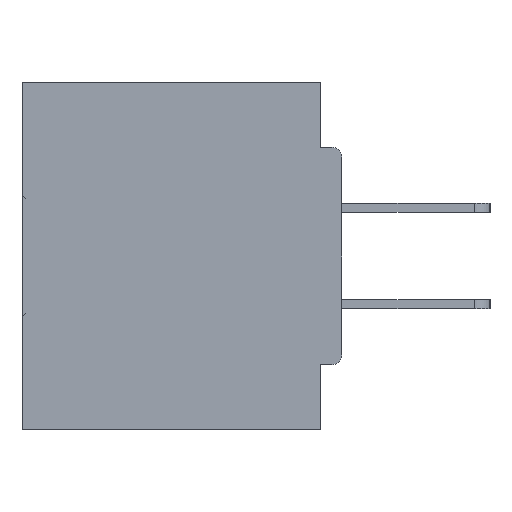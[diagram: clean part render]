
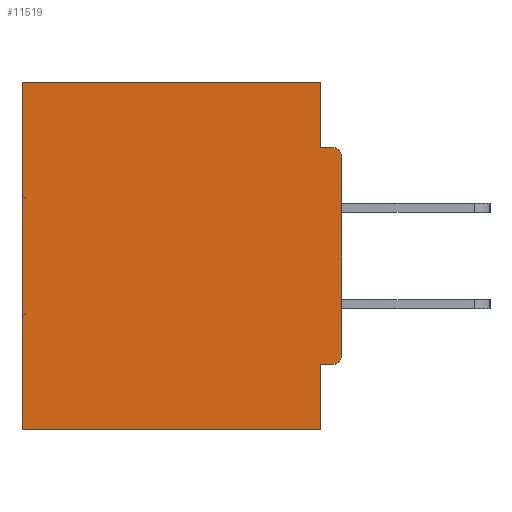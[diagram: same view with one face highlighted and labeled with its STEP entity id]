
A CAD part, left-side view. The second image highlights one B-rep face of the part: STEP entity #11519.
In plain terms, the highlighted planar face has unit normal (-1, 0, 0).
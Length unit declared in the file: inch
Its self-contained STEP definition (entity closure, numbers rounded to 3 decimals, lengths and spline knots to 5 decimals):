
#650 = DIRECTION ( 'NONE',  ( 0., 0., -1. ) ) ;
#1674 = CARTESIAN_POINT ( 'NONE',  ( 0.298, 0.031, -0.5 ) ) ;
#2309 = DIRECTION ( 'NONE',  ( 0., 0., -1. ) ) ;
#2411 = CARTESIAN_POINT ( 'NONE',  ( 0.298, 0.031, -0.5 ) ) ;
#2700 = VECTOR ( 'NONE', #34223, 39.37008 ) ;
#2734 = EDGE_CURVE ( 'NONE', #3310, #17542, #43901, .T. ) ;
#2821 = VECTOR ( 'NONE', #18981, 39.37008 ) ;
#2881 = ORIENTED_EDGE ( 'NONE', *, *, #22470, .F. ) ;
#3310 = VERTEX_POINT ( 'NONE', #43236 ) ;
#4273 = VERTEX_POINT ( 'NONE', #42371 ) ;
#4668 = ORIENTED_EDGE ( 'NONE', *, *, #32894, .F. ) ;
#4738 = VECTOR ( 'NONE', #2309, 39.37008 ) ;
#4815 = CARTESIAN_POINT ( 'NONE',  ( 0.298, 0., 0. ) ) ;
#5867 = CIRCLE ( 'NONE', #31879, 0.015 ) ;
#6453 = ORIENTED_EDGE ( 'NONE', *, *, #44425, .F. ) ;
#6900 = LINE ( 'NONE', #30315, #4738 ) ;
#7032 = DIRECTION ( 'NONE',  ( 0., 0., -1. ) ) ;
#7067 = CARTESIAN_POINT ( 'NONE',  ( 0.298, 0., -0.0935 ) ) ;
#7147 = VERTEX_POINT ( 'NONE', #1674 ) ;
#8447 = DIRECTION ( 'NONE',  ( 0., 0., -1. ) ) ;
#9360 = EDGE_CURVE ( 'NONE', #7147, #17542, #41419, .T. ) ;
#10008 = CARTESIAN_POINT ( 'NONE',  ( 0.298, 0., -0.3915 ) ) ;
#10308 = CARTESIAN_POINT ( 'NONE',  ( 0.298, 0.46, -0.5 ) ) ;
#10329 = CARTESIAN_POINT ( 'NONE',  ( 0.298, 0.015, -0.4065 ) ) ;
#10981 = VERTEX_POINT ( 'NONE', #10329 ) ;
#11519 = ADVANCED_FACE ( 'NONE', ( #39251 ), #18842, .F. ) ;
#11791 = CARTESIAN_POINT ( 'NONE',  ( 0.298, 0.015, -0.1085 ) ) ;
#11940 = EDGE_CURVE ( 'NONE', #10981, #24321, #34385, .T. ) ;
#13365 = DIRECTION ( 'NONE',  ( 0., 1., 0. ) ) ;
#14458 = ORIENTED_EDGE ( 'NONE', *, *, #2734, .T. ) ;
#15393 = ORIENTED_EDGE ( 'NONE', *, *, #26734, .F. ) ;
#15981 = ORIENTED_EDGE ( 'NONE', *, *, #9360, .F. ) ;
#16118 = AXIS2_PLACEMENT_3D ( 'NONE', #21905, #42683, #29031 ) ;
#16485 = CARTESIAN_POINT ( 'NONE',  ( 0.298, 0.031, -0.0935 ) ) ;
#17542 = VERTEX_POINT ( 'NONE', #10308 ) ;
#18842 = PLANE ( 'NONE',  #16118 ) ;
#18981 = DIRECTION ( 'NONE',  ( 0., 1., 0. ) ) ;
#21098 = DIRECTION ( 'NONE',  ( 0., -1., 0. ) ) ;
#21227 = LINE ( 'NONE', #2411, #2700 ) ;
#21905 = CARTESIAN_POINT ( 'NONE',  ( 0.298, 0., 0. ) ) ;
#22470 = EDGE_CURVE ( 'NONE', #24321, #7147, #21227, .T. ) ;
#22751 = DIRECTION ( 'NONE',  ( 0., 1., 0. ) ) ;
#22793 = VECTOR ( 'NONE', #21098, 39.37008 ) ;
#23067 = CARTESIAN_POINT ( 'NONE',  ( 0.298, 0., -0.5 ) ) ;
#23144 = EDGE_CURVE ( 'NONE', #32583, #4273, #37032, .T. ) ;
#24321 = VERTEX_POINT ( 'NONE', #33724 ) ;
#24850 = CARTESIAN_POINT ( 'NONE',  ( 0.298, 0.46, 0. ) ) ;
#25081 = VECTOR ( 'NONE', #13365, 39.37008 ) ;
#25689 = VECTOR ( 'NONE', #22751, 39.37008 ) ;
#26417 = DIRECTION ( 'NONE',  ( -1., 0., 0. ) ) ;
#26734 = EDGE_CURVE ( 'NONE', #43732, #31339, #6900, .T. ) ;
#27006 = VECTOR ( 'NONE', #650, 39.37008 ) ;
#27881 = ORIENTED_EDGE ( 'NONE', *, *, #41100, .T. ) ;
#29031 = DIRECTION ( 'NONE',  ( 0., 0., -1. ) ) ;
#30315 = CARTESIAN_POINT ( 'NONE',  ( 0.298, 0.031, -0.5 ) ) ;
#31339 = VERTEX_POINT ( 'NONE', #16485 ) ;
#31353 = AXIS2_PLACEMENT_3D ( 'NONE', #11791, #36349, #36644 ) ;
#31879 = AXIS2_PLACEMENT_3D ( 'NONE', #36483, #26417, #8447 ) ;
#32151 = CARTESIAN_POINT ( 'NONE',  ( 0.298, 0., -0.1085 ) ) ;
#32583 = VERTEX_POINT ( 'NONE', #32151 ) ;
#32894 = EDGE_CURVE ( 'NONE', #31339, #4273, #37480, .T. ) ;
#33724 = CARTESIAN_POINT ( 'NONE',  ( 0.298, 0.031, -0.4065 ) ) ;
#34097 = ORIENTED_EDGE ( 'NONE', *, *, #38607, .T. ) ;
#34223 = DIRECTION ( 'NONE',  ( 0., 0., -1. ) ) ;
#34293 = ORIENTED_EDGE ( 'NONE', *, *, #11940, .F. ) ;
#34385 = LINE ( 'NONE', #34865, #25081 ) ;
#34865 = CARTESIAN_POINT ( 'NONE',  ( 0.298, 0., -0.4065 ) ) ;
#35260 = VECTOR ( 'NONE', #7032, 39.37008 ) ;
#35821 = CARTESIAN_POINT ( 'NONE',  ( 0.298, 0., 0. ) ) ;
#35896 = ORIENTED_EDGE ( 'NONE', *, *, #23144, .T. ) ;
#36272 = LINE ( 'NONE', #35821, #27006 ) ;
#36349 = DIRECTION ( 'NONE',  ( -1., 0., 0. ) ) ;
#36483 = CARTESIAN_POINT ( 'NONE',  ( 0.298, 0.015, -0.3915 ) ) ;
#36577 = LINE ( 'NONE', #4815, #2821 ) ;
#36644 = DIRECTION ( 'NONE',  ( 0., 0., -1. ) ) ;
#37032 = CIRCLE ( 'NONE', #31353, 0.015 ) ;
#37480 = LINE ( 'NONE', #7067, #22793 ) ;
#38607 = EDGE_CURVE ( 'NONE', #43732, #3310, #36577, .T. ) ;
#39251 = FACE_OUTER_BOUND ( 'NONE', #44409, .T. ) ;
#41100 = EDGE_CURVE ( 'NONE', #10981, #41667, #5867, .T. ) ;
#41197 = CARTESIAN_POINT ( 'NONE',  ( 0.298, 0.031, 0. ) ) ;
#41419 = LINE ( 'NONE', #23067, #25689 ) ;
#41667 = VERTEX_POINT ( 'NONE', #10008 ) ;
#42371 = CARTESIAN_POINT ( 'NONE',  ( 0.298, 0.015, -0.0935 ) ) ;
#42683 = DIRECTION ( 'NONE',  ( 1., 0., 0. ) ) ;
#43236 = CARTESIAN_POINT ( 'NONE',  ( 0.298, 0.46, 0. ) ) ;
#43732 = VERTEX_POINT ( 'NONE', #41197 ) ;
#43901 = LINE ( 'NONE', #24850, #35260 ) ;
#44409 = EDGE_LOOP ( 'NONE', ( #35896, #4668, #15393, #34097, #14458, #15981, #2881, #34293, #27881, #6453 ) ) ;
#44425 = EDGE_CURVE ( 'NONE', #32583, #41667, #36272, .T. ) ;
